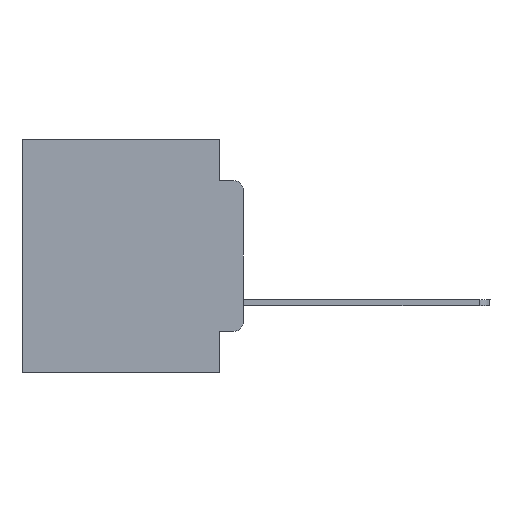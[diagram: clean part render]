
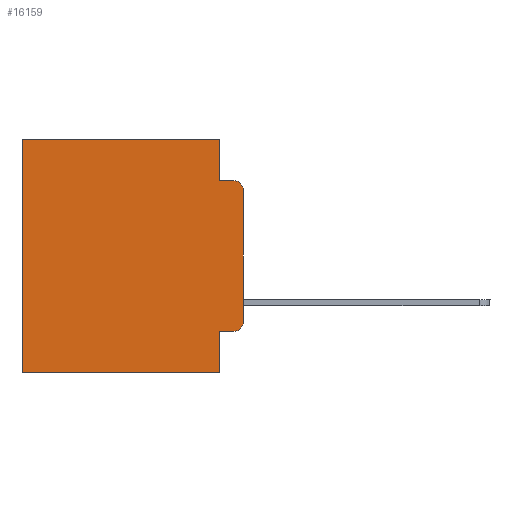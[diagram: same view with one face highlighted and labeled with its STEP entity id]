
A CAD part, left-side view. The second image highlights one B-rep face of the part: STEP entity #16159.
In plain terms, the highlighted planar face has unit normal (-1, 0, 0).
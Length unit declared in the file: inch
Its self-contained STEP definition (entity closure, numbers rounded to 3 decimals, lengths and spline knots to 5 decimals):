
#87 = ORIENTED_EDGE ( 'NONE', *, *, #7452, .T. ) ;
#639 = EDGE_CURVE ( 'NONE', #14344, #24878, #21543, .T. ) ;
#867 = DIRECTION ( 'NONE',  ( 0., -1., 0. ) ) ;
#985 = VERTEX_POINT ( 'NONE', #10045 ) ;
#1498 = CIRCLE ( 'NONE', #11526, 0.02 ) ;
#1560 = EDGE_CURVE ( 'NONE', #16104, #985, #10891, .T. ) ;
#3125 = DIRECTION ( 'NONE',  ( -1., 0., 0. ) ) ;
#3345 = CARTESIAN_POINT ( 'NONE',  ( 0.298, 0.051, -0.4115 ) ) ;
#3609 = CARTESIAN_POINT ( 'NONE',  ( 0.298, 0.051, -0.4115 ) ) ;
#4115 = CARTESIAN_POINT ( 'NONE',  ( 0.298, 0., -0.1085 ) ) ;
#4786 = VECTOR ( 'NONE', #11009, 39.37008 ) ;
#5841 = VERTEX_POINT ( 'NONE', #13350 ) ;
#6177 = EDGE_CURVE ( 'NONE', #16104, #6574, #19280, .T. ) ;
#6190 = VECTOR ( 'NONE', #19896, 39.37008 ) ;
#6285 = FACE_OUTER_BOUND ( 'NONE', #12900, .T. ) ;
#6413 = DIRECTION ( 'NONE',  ( 0., 0., -1. ) ) ;
#6507 = VERTEX_POINT ( 'NONE', #22554 ) ;
#6542 = LINE ( 'NONE', #20672, #10048 ) ;
#6574 = VERTEX_POINT ( 'NONE', #21425 ) ;
#7061 = CARTESIAN_POINT ( 'NONE',  ( 0.298, 0., -0.5 ) ) ;
#7258 = VERTEX_POINT ( 'NONE', #22998 ) ;
#7452 = EDGE_CURVE ( 'NONE', #24878, #6574, #1498, .T. ) ;
#7606 = DIRECTION ( 'NONE',  ( 0., 1., 0. ) ) ;
#7792 = CARTESIAN_POINT ( 'NONE',  ( 0.298, 0.02, -0.1085 ) ) ;
#7825 = CARTESIAN_POINT ( 'NONE',  ( 0.298, 0.051, 0. ) ) ;
#8026 = CARTESIAN_POINT ( 'NONE',  ( 0.298, 0.473, 0. ) ) ;
#8106 = AXIS2_PLACEMENT_3D ( 'NONE', #24793, #20812, #10372 ) ;
#8358 = ORIENTED_EDGE ( 'NONE', *, *, #1560, .T. ) ;
#8550 = VECTOR ( 'NONE', #21699, 39.37008 ) ;
#8717 = AXIS2_PLACEMENT_3D ( 'NONE', #7792, #18503, #13907 ) ;
#8935 = VECTOR ( 'NONE', #7606, 39.37008 ) ;
#8943 = LINE ( 'NONE', #9077, #8550 ) ;
#9077 = CARTESIAN_POINT ( 'NONE',  ( 0.298, 0.051, -0.0885 ) ) ;
#9395 = DIRECTION ( 'NONE',  ( 0., 0., -1. ) ) ;
#9415 = ORIENTED_EDGE ( 'NONE', *, *, #11345, .F. ) ;
#10045 = CARTESIAN_POINT ( 'NONE',  ( 0.298, 0.02, -0.0885 ) ) ;
#10048 = VECTOR ( 'NONE', #6413, 39.37008 ) ;
#10372 = DIRECTION ( 'NONE',  ( 0., 0., -1. ) ) ;
#10459 = CARTESIAN_POINT ( 'NONE',  ( 0.298, 0.473, 0. ) ) ;
#10891 = CIRCLE ( 'NONE', #8717, 0.02 ) ;
#11009 = DIRECTION ( 'NONE',  ( 0., 0., -1. ) ) ;
#11282 = DIRECTION ( 'NONE',  ( 0., 1., 0. ) ) ;
#11345 = EDGE_CURVE ( 'NONE', #16406, #7258, #19758, .T. ) ;
#11526 = AXIS2_PLACEMENT_3D ( 'NONE', #21744, #3125, #9395 ) ;
#11625 = VECTOR ( 'NONE', #867, 39.37008 ) ;
#12900 = EDGE_LOOP ( 'NONE', ( #16756, #8358, #20041, #9415, #15734, #21349, #16502, #24019, #25583, #87 ) ) ;
#13177 = CARTESIAN_POINT ( 'NONE',  ( 0.298, 0., 0. ) ) ;
#13350 = CARTESIAN_POINT ( 'NONE',  ( 0.298, 0.473, -0.5 ) ) ;
#13462 = LINE ( 'NONE', #7061, #16260 ) ;
#13907 = DIRECTION ( 'NONE',  ( 0., 0., -1. ) ) ;
#13984 = EDGE_CURVE ( 'NONE', #16406, #18840, #18193, .T. ) ;
#14344 = VERTEX_POINT ( 'NONE', #3609 ) ;
#15734 = ORIENTED_EDGE ( 'NONE', *, *, #13984, .T. ) ;
#16104 = VERTEX_POINT ( 'NONE', #4115 ) ;
#16159 = ADVANCED_FACE ( 'NONE', ( #6285 ), #20413, .F. ) ;
#16260 = VECTOR ( 'NONE', #11282, 39.37008 ) ;
#16406 = VERTEX_POINT ( 'NONE', #21914 ) ;
#16502 = ORIENTED_EDGE ( 'NONE', *, *, #24791, .F. ) ;
#16719 = EDGE_CURVE ( 'NONE', #7258, #985, #8943, .T. ) ;
#16756 = ORIENTED_EDGE ( 'NONE', *, *, #6177, .F. ) ;
#17457 = EDGE_CURVE ( 'NONE', #18840, #5841, #26655, .T. ) ;
#18193 = LINE ( 'NONE', #24456, #8935 ) ;
#18503 = DIRECTION ( 'NONE',  ( -1., 0., 0. ) ) ;
#18840 = VERTEX_POINT ( 'NONE', #10459 ) ;
#19280 = LINE ( 'NONE', #13177, #4786 ) ;
#19758 = LINE ( 'NONE', #7825, #6190 ) ;
#19896 = DIRECTION ( 'NONE',  ( 0., 0., -1. ) ) ;
#20041 = ORIENTED_EDGE ( 'NONE', *, *, #16719, .F. ) ;
#20413 = PLANE ( 'NONE',  #8106 ) ;
#20672 = CARTESIAN_POINT ( 'NONE',  ( 0.298, 0.051, 0. ) ) ;
#20812 = DIRECTION ( 'NONE',  ( 1., 0., 0. ) ) ;
#21349 = ORIENTED_EDGE ( 'NONE', *, *, #17457, .T. ) ;
#21425 = CARTESIAN_POINT ( 'NONE',  ( 0.298, 0., -0.3915 ) ) ;
#21543 = LINE ( 'NONE', #3345, #11625 ) ;
#21698 = EDGE_CURVE ( 'NONE', #14344, #6507, #6542, .T. ) ;
#21699 = DIRECTION ( 'NONE',  ( 0., -1., 0. ) ) ;
#21744 = CARTESIAN_POINT ( 'NONE',  ( 0.298, 0.02, -0.3915 ) ) ;
#21914 = CARTESIAN_POINT ( 'NONE',  ( 0.298, 0.051, 0. ) ) ;
#22554 = CARTESIAN_POINT ( 'NONE',  ( 0.298, 0.051, -0.5 ) ) ;
#22998 = CARTESIAN_POINT ( 'NONE',  ( 0.298, 0.051, -0.0885 ) ) ;
#24019 = ORIENTED_EDGE ( 'NONE', *, *, #21698, .F. ) ;
#24077 = CARTESIAN_POINT ( 'NONE',  ( 0.298, 0.02, -0.4115 ) ) ;
#24456 = CARTESIAN_POINT ( 'NONE',  ( 0.298, 0., 0. ) ) ;
#24619 = DIRECTION ( 'NONE',  ( 0., 0., -1. ) ) ;
#24791 = EDGE_CURVE ( 'NONE', #6507, #5841, #13462, .T. ) ;
#24793 = CARTESIAN_POINT ( 'NONE',  ( 0.298, 0., 0. ) ) ;
#24878 = VERTEX_POINT ( 'NONE', #24077 ) ;
#25518 = VECTOR ( 'NONE', #24619, 39.37008 ) ;
#25583 = ORIENTED_EDGE ( 'NONE', *, *, #639, .T. ) ;
#26655 = LINE ( 'NONE', #8026, #25518 ) ;
